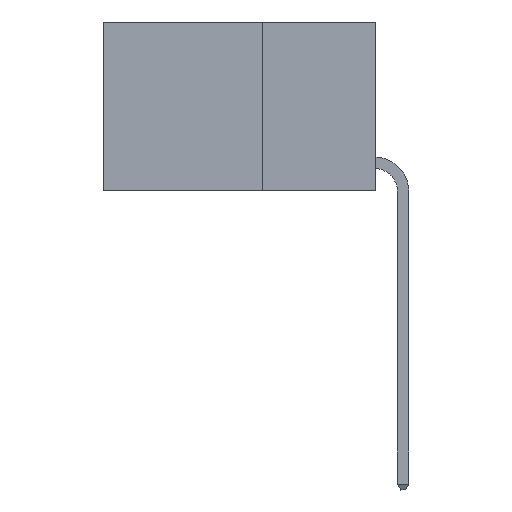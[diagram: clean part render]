
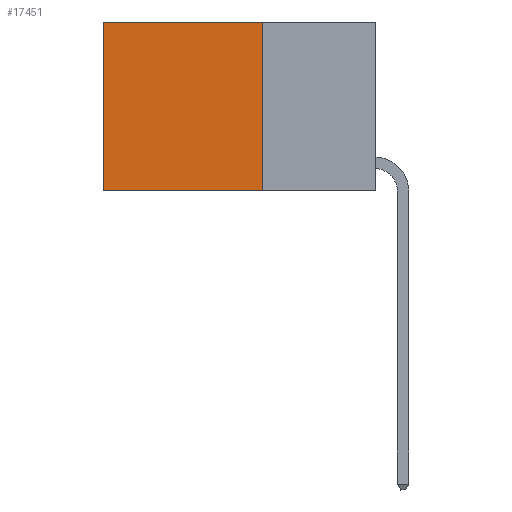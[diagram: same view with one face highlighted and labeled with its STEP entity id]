
A CAD part, left-side view. The second image highlights one B-rep face of the part: STEP entity #17451.
In plain terms, the highlighted planar face has unit normal (-1, 0, 0).
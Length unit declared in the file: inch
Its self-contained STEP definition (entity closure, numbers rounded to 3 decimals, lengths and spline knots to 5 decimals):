
#93 = DIRECTION ( 'NONE',  ( 0., 1., 0. ) ) ;
#121 = CARTESIAN_POINT ( 'NONE',  ( 0.2625, 0.6, 0. ) ) ;
#327 = DIRECTION ( 'NONE',  ( 0., 0., -1. ) ) ;
#360 = CARTESIAN_POINT ( 'NONE',  ( 0.2625, 0.6, 0. ) ) ;
#1680 = DIRECTION ( 'NONE',  ( 1., 0., 0. ) ) ;
#1813 = VECTOR ( 'NONE', #93, 39.37008 ) ;
#2078 = LINE ( 'NONE', #12313, #13284 ) ;
#2091 = VERTEX_POINT ( 'NONE', #9599 ) ;
#2128 = CARTESIAN_POINT ( 'NONE',  ( 0.2625, 0.25, 0. ) ) ;
#2221 = PLANE ( 'NONE',  #15437 ) ;
#2228 = ORIENTED_EDGE ( 'NONE', *, *, #17020, .F. ) ;
#3450 = LINE ( 'NONE', #7690, #5290 ) ;
#4765 = ORIENTED_EDGE ( 'NONE', *, *, #10018, .T. ) ;
#4804 = VECTOR ( 'NONE', #14913, 39.37008 ) ;
#5290 = VECTOR ( 'NONE', #12317, 39.37008 ) ;
#6314 = LINE ( 'NONE', #121, #4804 ) ;
#7690 = CARTESIAN_POINT ( 'NONE',  ( 0.2625, 0.25, -0.37 ) ) ;
#7696 = VERTEX_POINT ( 'NONE', #13219 ) ;
#9599 = CARTESIAN_POINT ( 'NONE',  ( 0.2625, 0.25, 0. ) ) ;
#10018 = EDGE_CURVE ( 'NONE', #10386, #14204, #6314, .T. ) ;
#10386 = VERTEX_POINT ( 'NONE', #360 ) ;
#11112 = DIRECTION ( 'NONE',  ( 0., 0., -1. ) ) ;
#12313 = CARTESIAN_POINT ( 'NONE',  ( 0.2625, 0.25, 0. ) ) ;
#12317 = DIRECTION ( 'NONE',  ( 0., 1., 0. ) ) ;
#12590 = EDGE_LOOP ( 'NONE', ( #4765, #17861, #2228, #13093 ) ) ;
#12967 = CARTESIAN_POINT ( 'NONE',  ( 0.2625, 0.6, -0.37 ) ) ;
#13093 = ORIENTED_EDGE ( 'NONE', *, *, #15883, .T. ) ;
#13219 = CARTESIAN_POINT ( 'NONE',  ( 0.2625, 0.25, -0.37 ) ) ;
#13284 = VECTOR ( 'NONE', #327, 39.37008 ) ;
#13526 = CARTESIAN_POINT ( 'NONE',  ( 0.2625, 0.25, 0. ) ) ;
#14119 = LINE ( 'NONE', #13526, #1813 ) ;
#14204 = VERTEX_POINT ( 'NONE', #12967 ) ;
#14913 = DIRECTION ( 'NONE',  ( 0., 0., -1. ) ) ;
#15437 = AXIS2_PLACEMENT_3D ( 'NONE', #2128, #1680, #11112 ) ;
#15883 = EDGE_CURVE ( 'NONE', #2091, #10386, #14119, .T. ) ;
#17020 = EDGE_CURVE ( 'NONE', #2091, #7696, #2078, .T. ) ;
#17451 = ADVANCED_FACE ( 'NONE', ( #18436 ), #2221, .F. ) ;
#17861 = ORIENTED_EDGE ( 'NONE', *, *, #18344, .F. ) ;
#18344 = EDGE_CURVE ( 'NONE', #7696, #14204, #3450, .T. ) ;
#18436 = FACE_OUTER_BOUND ( 'NONE', #12590, .T. ) ;
